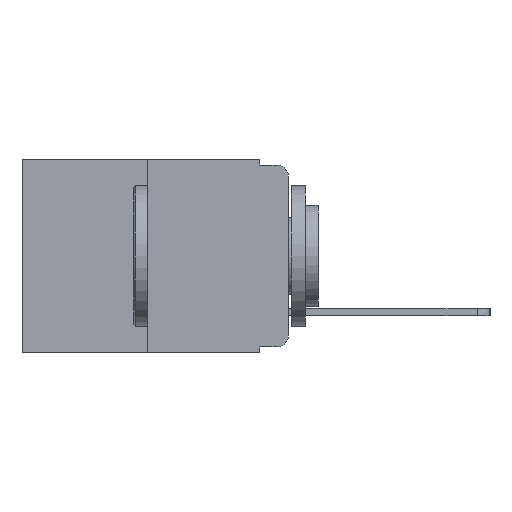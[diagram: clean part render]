
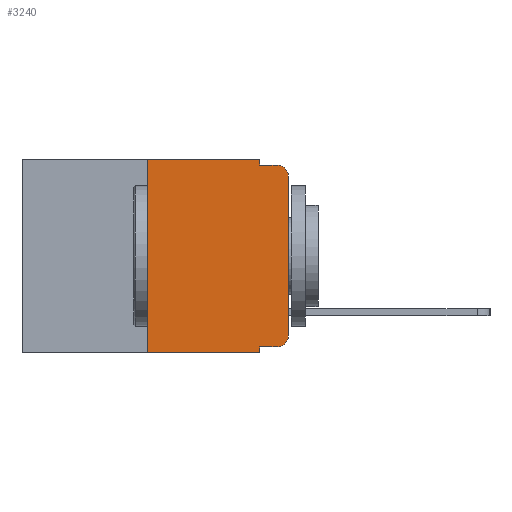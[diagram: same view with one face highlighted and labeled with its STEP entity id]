
A CAD part, left-side view. The second image highlights one B-rep face of the part: STEP entity #3240.
In plain terms, the highlighted planar face has unit normal (-1, 0, 0).
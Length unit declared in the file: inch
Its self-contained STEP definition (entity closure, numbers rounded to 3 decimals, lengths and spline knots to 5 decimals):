
#360 = EDGE_LOOP ( 'NONE', ( #3181, #8251, #879, #8547, #11115, #1182, #3788, #8847, #1488, #4094 ) ) ;
#533 = CARTESIAN_POINT ( 'NONE',  ( 0., 0., -0.313 ) ) ;
#754 = CARTESIAN_POINT ( 'NONE',  ( 0., 0.25, -0.343 ) ) ;
#879 = ORIENTED_EDGE ( 'NONE', *, *, #7728, .F. ) ;
#1097 = LINE ( 'NONE', #7357, #8459 ) ;
#1182 = ORIENTED_EDGE ( 'NONE', *, *, #6458, .F. ) ;
#1348 = VECTOR ( 'NONE', #11846, 39.37008 ) ;
#1488 = ORIENTED_EDGE ( 'NONE', *, *, #5165, .T. ) ;
#1690 = DIRECTION ( 'NONE',  ( 0., -1., 0. ) ) ;
#1818 = VECTOR ( 'NONE', #11161, 39.37008 ) ;
#1918 = CARTESIAN_POINT ( 'NONE',  ( 0., 0.051, 0. ) ) ;
#1935 = CARTESIAN_POINT ( 'NONE',  ( 0., 0.051, -0.343 ) ) ;
#2342 = VERTEX_POINT ( 'NONE', #1918 ) ;
#2468 = VECTOR ( 'NONE', #6396, 39.37008 ) ;
#2509 = VERTEX_POINT ( 'NONE', #533 ) ;
#2773 = CARTESIAN_POINT ( 'NONE',  ( 0., 0., 0. ) ) ;
#2889 = CARTESIAN_POINT ( 'NONE',  ( 0., 0.25, 0. ) ) ;
#2905 = VERTEX_POINT ( 'NONE', #7349 ) ;
#3092 = CIRCLE ( 'NONE', #7161, 0.02 ) ;
#3181 = ORIENTED_EDGE ( 'NONE', *, *, #9628, .T. ) ;
#3231 = CARTESIAN_POINT ( 'NONE',  ( 0., 0.02, -0.313 ) ) ;
#3240 = ADVANCED_FACE ( 'NONE', ( #9545 ), #10338, .F. ) ;
#3271 = CARTESIAN_POINT ( 'NONE',  ( 0., 0., -0.03 ) ) ;
#3788 = ORIENTED_EDGE ( 'NONE', *, *, #11489, .T. ) ;
#4094 = ORIENTED_EDGE ( 'NONE', *, *, #4523, .T. ) ;
#4195 = DIRECTION ( 'NONE',  ( 0., 0., -1. ) ) ;
#4289 = VECTOR ( 'NONE', #10437, 39.37008 ) ;
#4308 = VERTEX_POINT ( 'NONE', #6829 ) ;
#4523 = EDGE_CURVE ( 'NONE', #2905, #2509, #3092, .T. ) ;
#4583 = DIRECTION ( 'NONE',  ( -1., 0., 0. ) ) ;
#4667 = VERTEX_POINT ( 'NONE', #11985 ) ;
#5165 = EDGE_CURVE ( 'NONE', #6472, #2905, #1097, .T. ) ;
#5417 = CARTESIAN_POINT ( 'NONE',  ( 0., 0.051, -0.333 ) ) ;
#5824 = EDGE_CURVE ( 'NONE', #6472, #6722, #7280, .T. ) ;
#6396 = DIRECTION ( 'NONE',  ( 0., 0., -1. ) ) ;
#6458 = EDGE_CURVE ( 'NONE', #9591, #10372, #11534, .T. ) ;
#6471 = VECTOR ( 'NONE', #11081, 39.37008 ) ;
#6472 = VERTEX_POINT ( 'NONE', #5417 ) ;
#6524 = LINE ( 'NONE', #10894, #1348 ) ;
#6722 = VERTEX_POINT ( 'NONE', #1935 ) ;
#6829 = CARTESIAN_POINT ( 'NONE',  ( 0., 0.051, -0.01 ) ) ;
#6907 = LINE ( 'NONE', #9388, #11655 ) ;
#7092 = EDGE_CURVE ( 'NONE', #2342, #4308, #6907, .T. ) ;
#7161 = AXIS2_PLACEMENT_3D ( 'NONE', #3231, #9924, #4195 ) ;
#7280 = LINE ( 'NONE', #10214, #2468 ) ;
#7284 = CARTESIAN_POINT ( 'NONE',  ( 0., 0.25, 0. ) ) ;
#7349 = CARTESIAN_POINT ( 'NONE',  ( 0., 0.02, -0.333 ) ) ;
#7357 = CARTESIAN_POINT ( 'NONE',  ( 0., 0.051, -0.333 ) ) ;
#7728 = EDGE_CURVE ( 'NONE', #4308, #4667, #7902, .T. ) ;
#7902 = LINE ( 'NONE', #8402, #10153 ) ;
#8173 = CARTESIAN_POINT ( 'NONE',  ( 0., 0.473, 0. ) ) ;
#8251 = ORIENTED_EDGE ( 'NONE', *, *, #8334, .T. ) ;
#8288 = DIRECTION ( 'NONE',  ( 0., -1., 0. ) ) ;
#8334 = EDGE_CURVE ( 'NONE', #9964, #4667, #11054, .T. ) ;
#8402 = CARTESIAN_POINT ( 'NONE',  ( 0., 0.051, -0.01 ) ) ;
#8459 = VECTOR ( 'NONE', #8288, 39.37008 ) ;
#8547 = ORIENTED_EDGE ( 'NONE', *, *, #7092, .F. ) ;
#8549 = AXIS2_PLACEMENT_3D ( 'NONE', #8173, #10315, #10275 ) ;
#8847 = ORIENTED_EDGE ( 'NONE', *, *, #5824, .F. ) ;
#9217 = CARTESIAN_POINT ( 'NONE',  ( 0., 0.473, 0. ) ) ;
#9368 = LINE ( 'NONE', #2773, #4289 ) ;
#9388 = CARTESIAN_POINT ( 'NONE',  ( 0., 0.051, 0. ) ) ;
#9426 = DIRECTION ( 'NONE',  ( 0., 0., -1. ) ) ;
#9545 = FACE_OUTER_BOUND ( 'NONE', #360, .T. ) ;
#9591 = VERTEX_POINT ( 'NONE', #754 ) ;
#9628 = EDGE_CURVE ( 'NONE', #2509, #9964, #9368, .T. ) ;
#9924 = DIRECTION ( 'NONE',  ( -1., 0., 0. ) ) ;
#9964 = VERTEX_POINT ( 'NONE', #3271 ) ;
#10153 = VECTOR ( 'NONE', #1690, 39.37008 ) ;
#10214 = CARTESIAN_POINT ( 'NONE',  ( 0., 0.051, 0. ) ) ;
#10275 = DIRECTION ( 'NONE',  ( 0., 0., -1. ) ) ;
#10288 = CARTESIAN_POINT ( 'NONE',  ( 0., 0.02, -0.03 ) ) ;
#10315 = DIRECTION ( 'NONE',  ( 1., 0., 0. ) ) ;
#10338 = PLANE ( 'NONE',  #8549 ) ;
#10372 = VERTEX_POINT ( 'NONE', #2889 ) ;
#10437 = DIRECTION ( 'NONE',  ( 0., 0., 1. ) ) ;
#10894 = CARTESIAN_POINT ( 'NONE',  ( 0., 0.473, -0.343 ) ) ;
#11054 = CIRCLE ( 'NONE', #12349, 0.02 ) ;
#11081 = DIRECTION ( 'NONE',  ( 0., 0., 1. ) ) ;
#11115 = ORIENTED_EDGE ( 'NONE', *, *, #11648, .F. ) ;
#11161 = DIRECTION ( 'NONE',  ( 0., -1., 0. ) ) ;
#11264 = DIRECTION ( 'NONE',  ( 0., 0., -1. ) ) ;
#11489 = EDGE_CURVE ( 'NONE', #9591, #6722, #6524, .T. ) ;
#11534 = LINE ( 'NONE', #7284, #6471 ) ;
#11648 = EDGE_CURVE ( 'NONE', #10372, #2342, #11994, .T. ) ;
#11655 = VECTOR ( 'NONE', #9426, 39.37008 ) ;
#11846 = DIRECTION ( 'NONE',  ( 0., -1., 0. ) ) ;
#11985 = CARTESIAN_POINT ( 'NONE',  ( 0., 0.02, -0.01 ) ) ;
#11994 = LINE ( 'NONE', #9217, #1818 ) ;
#12349 = AXIS2_PLACEMENT_3D ( 'NONE', #10288, #4583, #11264 ) ;
